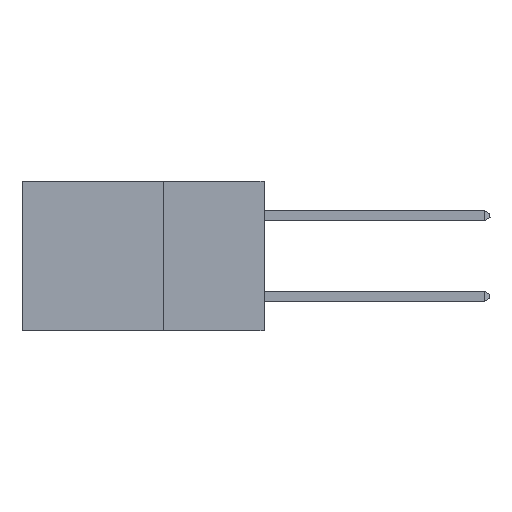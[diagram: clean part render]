
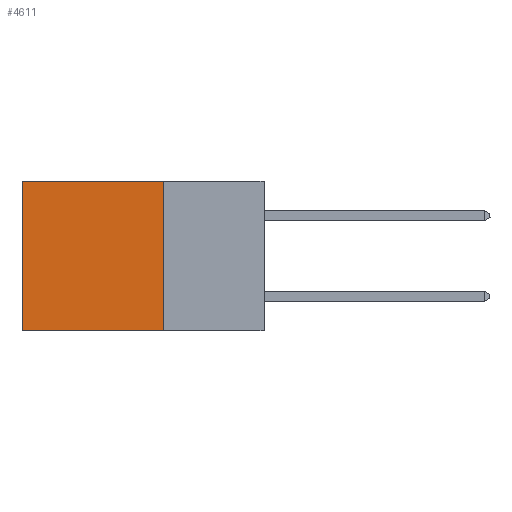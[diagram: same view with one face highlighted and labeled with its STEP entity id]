
A CAD part, left-side view. The second image highlights one B-rep face of the part: STEP entity #4611.
In plain terms, the highlighted planar face has unit normal (-1, 0, 0).
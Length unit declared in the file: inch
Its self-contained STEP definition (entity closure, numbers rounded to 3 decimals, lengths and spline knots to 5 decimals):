
#270 = EDGE_LOOP ( 'NONE', ( #10057, #5231, #960, #2219 ) ) ;
#751 = LINE ( 'NONE', #3255, #9190 ) ;
#830 = FACE_OUTER_BOUND ( 'NONE', #270, .T. ) ;
#960 = ORIENTED_EDGE ( 'NONE', *, *, #4005, .F. ) ;
#1213 = DIRECTION ( 'NONE',  ( 0., 1., 0. ) ) ;
#1872 = LINE ( 'NONE', #1944, #9413 ) ;
#1898 = LINE ( 'NONE', #2307, #10361 ) ;
#1944 = CARTESIAN_POINT ( 'NONE',  ( 0.298, 0.25, 0. ) ) ;
#2219 = ORIENTED_EDGE ( 'NONE', *, *, #9039, .T. ) ;
#2307 = CARTESIAN_POINT ( 'NONE',  ( 0.298, 0.25, 0. ) ) ;
#2400 = LINE ( 'NONE', #6609, #3034 ) ;
#2837 = EDGE_CURVE ( 'NONE', #7573, #5075, #2400, .T. ) ;
#3034 = VECTOR ( 'NONE', #4095, 39.37008 ) ;
#3255 = CARTESIAN_POINT ( 'NONE',  ( 0.298, 0.6, 0. ) ) ;
#3521 = DIRECTION ( 'NONE',  ( 1., 0., 0. ) ) ;
#4005 = EDGE_CURVE ( 'NONE', #9234, #7573, #1872, .T. ) ;
#4089 = AXIS2_PLACEMENT_3D ( 'NONE', #7583, #3521, #7610 ) ;
#4095 = DIRECTION ( 'NONE',  ( 0., 1., 0. ) ) ;
#4222 = CARTESIAN_POINT ( 'NONE',  ( 0.298, 0.25, 0. ) ) ;
#4611 = ADVANCED_FACE ( 'NONE', ( #830 ), #5378, .F. ) ;
#4906 = DIRECTION ( 'NONE',  ( 0., 0., -1. ) ) ;
#5075 = VERTEX_POINT ( 'NONE', #10509 ) ;
#5231 = ORIENTED_EDGE ( 'NONE', *, *, #2837, .F. ) ;
#5378 = PLANE ( 'NONE',  #4089 ) ;
#6609 = CARTESIAN_POINT ( 'NONE',  ( 0.298, 0.25, -0.37 ) ) ;
#7010 = DIRECTION ( 'NONE',  ( 0., 0., -1. ) ) ;
#7573 = VERTEX_POINT ( 'NONE', #9998 ) ;
#7583 = CARTESIAN_POINT ( 'NONE',  ( 0.298, 0.25, 0. ) ) ;
#7610 = DIRECTION ( 'NONE',  ( 0., 0., -1. ) ) ;
#9039 = EDGE_CURVE ( 'NONE', #9234, #9656, #1898, .T. ) ;
#9190 = VECTOR ( 'NONE', #4906, 39.37008 ) ;
#9234 = VERTEX_POINT ( 'NONE', #4222 ) ;
#9413 = VECTOR ( 'NONE', #7010, 39.37008 ) ;
#9625 = EDGE_CURVE ( 'NONE', #9656, #5075, #751, .T. ) ;
#9656 = VERTEX_POINT ( 'NONE', #9693 ) ;
#9693 = CARTESIAN_POINT ( 'NONE',  ( 0.298, 0.6, 0. ) ) ;
#9998 = CARTESIAN_POINT ( 'NONE',  ( 0.298, 0.25, -0.37 ) ) ;
#10057 = ORIENTED_EDGE ( 'NONE', *, *, #9625, .T. ) ;
#10361 = VECTOR ( 'NONE', #1213, 39.37008 ) ;
#10509 = CARTESIAN_POINT ( 'NONE',  ( 0.298, 0.6, -0.37 ) ) ;
